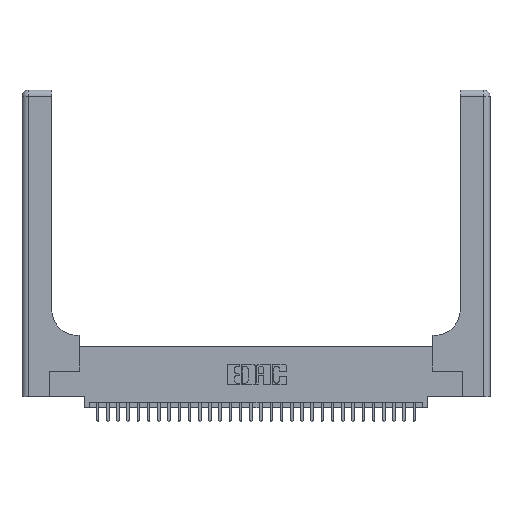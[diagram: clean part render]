
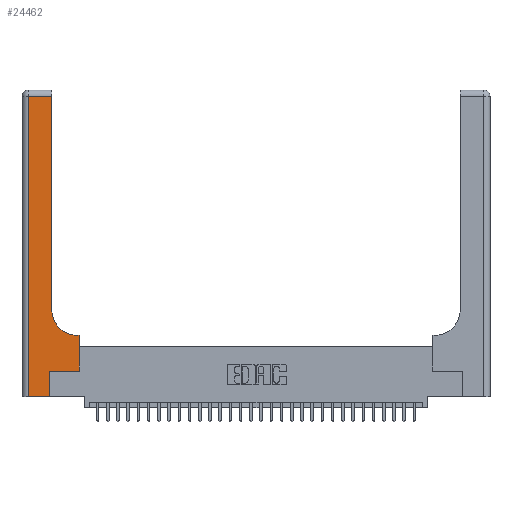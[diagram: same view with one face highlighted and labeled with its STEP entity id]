
A CAD part, top view. The second image highlights one B-rep face of the part: STEP entity #24462.
In plain terms, the highlighted planar face has unit normal (0, 0, 1).
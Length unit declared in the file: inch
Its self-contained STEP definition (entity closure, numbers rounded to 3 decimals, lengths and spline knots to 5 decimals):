
#83 = CARTESIAN_POINT ( 'NONE',  ( 0.5585, 0.25, 0.37 ) ) ;
#356 = CARTESIAN_POINT ( 'NONE',  ( 0., 0., 0.37 ) ) ;
#1460 = VECTOR ( 'NONE', #16836, 39.37008 ) ;
#1926 = EDGE_CURVE ( 'NONE', #10980, #3707, #9695, .T. ) ;
#2056 = LINE ( 'NONE', #31103, #20852 ) ;
#2226 = VERTEX_POINT ( 'NONE', #13138 ) ;
#3020 = AXIS2_PLACEMENT_3D ( 'NONE', #8481, #23079, #28118 ) ;
#3041 = VERTEX_POINT ( 'NONE', #28853 ) ;
#3153 = PLANE ( 'NONE',  #30894 ) ;
#3366 = DIRECTION ( 'NONE',  ( -1., 0., 0. ) ) ;
#3707 = VERTEX_POINT ( 'NONE', #21392 ) ;
#4353 = EDGE_CURVE ( 'NONE', #3707, #2226, #13396, .T. ) ;
#4783 = EDGE_CURVE ( 'NONE', #8782, #28100, #4926, .T. ) ;
#4913 = EDGE_CURVE ( 'NONE', #20465, #8782, #18354, .T. ) ;
#4926 = LINE ( 'NONE', #28539, #29128 ) ;
#5120 = EDGE_LOOP ( 'NONE', ( #23124, #25414, #8289, #10946, #8836, #13707, #6715, #9756, #30050 ) ) ;
#6068 = EDGE_CURVE ( 'NONE', #2226, #22699, #14051, .T. ) ;
#6125 = VECTOR ( 'NONE', #7308, 39.37008 ) ;
#6715 = ORIENTED_EDGE ( 'NONE', *, *, #1926, .T. ) ;
#6880 = CARTESIAN_POINT ( 'NONE',  ( 0.5585, 0.25, 0.37 ) ) ;
#7308 = DIRECTION ( 'NONE',  ( -1., 0., 0. ) ) ;
#7473 = LINE ( 'NONE', #7836, #13210 ) ;
#7836 = CARTESIAN_POINT ( 'NONE',  ( 0.269, 0., 0.37 ) ) ;
#8289 = ORIENTED_EDGE ( 'NONE', *, *, #4783, .T. ) ;
#8481 = CARTESIAN_POINT ( 'NONE',  ( 0.5415, 0.85, 0.37 ) ) ;
#8782 = VERTEX_POINT ( 'NONE', #31030 ) ;
#8836 = ORIENTED_EDGE ( 'NONE', *, *, #22539, .T. ) ;
#9441 = DIRECTION ( 'NONE',  ( 0., 1., 0. ) ) ;
#9511 = CARTESIAN_POINT ( 'NONE',  ( 0.2915, 3., 0.37 ) ) ;
#9695 = LINE ( 'NONE', #6880, #14658 ) ;
#9756 = ORIENTED_EDGE ( 'NONE', *, *, #4353, .T. ) ;
#9856 = CARTESIAN_POINT ( 'NONE',  ( 0.2915, 2.94, 0.37 ) ) ;
#10880 = FACE_OUTER_BOUND ( 'NONE', #5120, .T. ) ;
#10946 = ORIENTED_EDGE ( 'NONE', *, *, #15145, .T. ) ;
#10980 = VERTEX_POINT ( 'NONE', #83 ) ;
#13138 = CARTESIAN_POINT ( 'NONE',  ( 0.5415, 0.6, 0.37 ) ) ;
#13210 = VECTOR ( 'NONE', #15325, 39.37008 ) ;
#13396 = LINE ( 'NONE', #22203, #6125 ) ;
#13707 = ORIENTED_EDGE ( 'NONE', *, *, #24073, .T. ) ;
#14051 = CIRCLE ( 'NONE', #3020, 0.25 ) ;
#14353 = CARTESIAN_POINT ( 'NONE',  ( 0., 2.94, 0.37 ) ) ;
#14658 = VECTOR ( 'NONE', #9441, 39.37008 ) ;
#15145 = EDGE_CURVE ( 'NONE', #28100, #16905, #23740, .T. ) ;
#15153 = DIRECTION ( 'NONE',  ( 1., 0., 0. ) ) ;
#15325 = DIRECTION ( 'NONE',  ( 0., 1., 0. ) ) ;
#15799 = DIRECTION ( 'NONE',  ( 0., 0., -1. ) ) ;
#16836 = DIRECTION ( 'NONE',  ( -1., 0., 0. ) ) ;
#16905 = VERTEX_POINT ( 'NONE', #26346 ) ;
#17451 = VECTOR ( 'NONE', #24109, 39.37008 ) ;
#17935 = EDGE_CURVE ( 'NONE', #22699, #20465, #18571, .T. ) ;
#17993 = CARTESIAN_POINT ( 'NONE',  ( 0.06, 0., 0.37 ) ) ;
#18354 = LINE ( 'NONE', #14353, #1460 ) ;
#18571 = LINE ( 'NONE', #9511, #17451 ) ;
#20465 = VERTEX_POINT ( 'NONE', #9856 ) ;
#20852 = VECTOR ( 'NONE', #28736, 39.37008 ) ;
#21392 = CARTESIAN_POINT ( 'NONE',  ( 0.5585, 0.6, 0.37 ) ) ;
#22203 = CARTESIAN_POINT ( 'NONE',  ( 0.2915, 0.6, 0.37 ) ) ;
#22539 = EDGE_CURVE ( 'NONE', #16905, #3041, #7473, .T. ) ;
#22699 = VERTEX_POINT ( 'NONE', #23400 ) ;
#22780 = CARTESIAN_POINT ( 'NONE',  ( 0., 3., 0.37 ) ) ;
#23079 = DIRECTION ( 'NONE',  ( 0., 0., -1. ) ) ;
#23124 = ORIENTED_EDGE ( 'NONE', *, *, #17935, .T. ) ;
#23400 = CARTESIAN_POINT ( 'NONE',  ( 0.2915, 0.85, 0.37 ) ) ;
#23740 = LINE ( 'NONE', #356, #31813 ) ;
#24073 = EDGE_CURVE ( 'NONE', #3041, #10980, #2056, .T. ) ;
#24109 = DIRECTION ( 'NONE',  ( 0., 1., 0. ) ) ;
#24462 = ADVANCED_FACE ( 'NONE', ( #10880 ), #3153, .F. ) ;
#25414 = ORIENTED_EDGE ( 'NONE', *, *, #4913, .T. ) ;
#26346 = CARTESIAN_POINT ( 'NONE',  ( 0.269, 0., 0.37 ) ) ;
#28100 = VERTEX_POINT ( 'NONE', #17993 ) ;
#28118 = DIRECTION ( 'NONE',  ( 1., 0., 0. ) ) ;
#28539 = CARTESIAN_POINT ( 'NONE',  ( 0.06, 3., 0.37 ) ) ;
#28736 = DIRECTION ( 'NONE',  ( 1., 0., 0. ) ) ;
#28853 = CARTESIAN_POINT ( 'NONE',  ( 0.269, 0.25, 0.37 ) ) ;
#29128 = VECTOR ( 'NONE', #31343, 39.37008 ) ;
#30050 = ORIENTED_EDGE ( 'NONE', *, *, #6068, .T. ) ;
#30894 = AXIS2_PLACEMENT_3D ( 'NONE', #22780, #15799, #3366 ) ;
#31030 = CARTESIAN_POINT ( 'NONE',  ( 0.06, 2.94, 0.37 ) ) ;
#31103 = CARTESIAN_POINT ( 'NONE',  ( 0.269, 0.25, 0.37 ) ) ;
#31343 = DIRECTION ( 'NONE',  ( 0., -1., 0. ) ) ;
#31813 = VECTOR ( 'NONE', #15153, 39.37008 ) ;
